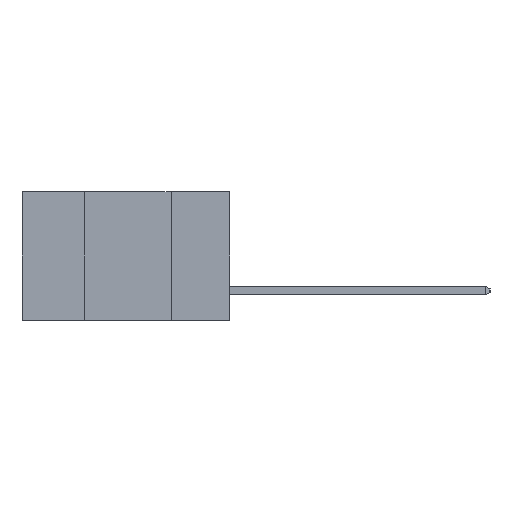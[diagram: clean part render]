
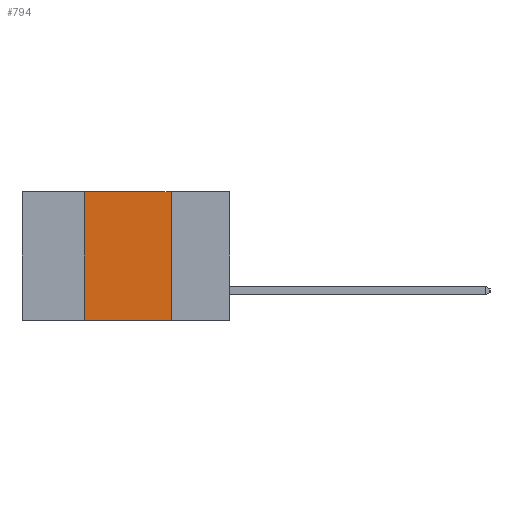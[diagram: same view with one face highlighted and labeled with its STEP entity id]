
A CAD part, left-side view. The second image highlights one B-rep face of the part: STEP entity #794.
In plain terms, the highlighted planar face has unit normal (-1, 0, 0).
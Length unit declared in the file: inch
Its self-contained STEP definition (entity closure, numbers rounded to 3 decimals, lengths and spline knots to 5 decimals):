
#26 = CARTESIAN_POINT ( 'NONE',  ( 0., 0.6, 0. ) ) ;
#627 = DIRECTION ( 'NONE',  ( 0., 0., -1. ) ) ;
#794 = ADVANCED_FACE ( 'NONE', ( #10889 ), #2431, .F. ) ;
#1288 = ORIENTED_EDGE ( 'NONE', *, *, #10157, .F. ) ;
#1415 = DIRECTION ( 'NONE',  ( 0., 0., 1. ) ) ;
#2431 = PLANE ( 'NONE',  #8279 ) ;
#2713 = LINE ( 'NONE', #5776, #10181 ) ;
#2920 = LINE ( 'NONE', #11767, #10082 ) ;
#3442 = VECTOR ( 'NONE', #8856, 39.37008 ) ;
#3503 = DIRECTION ( 'NONE',  ( 1., 0., 0. ) ) ;
#3769 = LINE ( 'NONE', #26, #3442 ) ;
#3923 = EDGE_LOOP ( 'NONE', ( #1288, #9534, #12179, #10366 ) ) ;
#3983 = VECTOR ( 'NONE', #1415, 39.37008 ) ;
#4303 = VERTEX_POINT ( 'NONE', #6328 ) ;
#4814 = CARTESIAN_POINT ( 'NONE',  ( 0., 0.6, 0. ) ) ;
#5368 = CARTESIAN_POINT ( 'NONE',  ( 0., 0.17, 0. ) ) ;
#5492 = VERTEX_POINT ( 'NONE', #7036 ) ;
#5776 = CARTESIAN_POINT ( 'NONE',  ( 0., 0.17, 0. ) ) ;
#6235 = LINE ( 'NONE', #7287, #3983 ) ;
#6251 = VERTEX_POINT ( 'NONE', #5368 ) ;
#6328 = CARTESIAN_POINT ( 'NONE',  ( 0., 0.42, -0.37 ) ) ;
#6390 = VERTEX_POINT ( 'NONE', #9241 ) ;
#6923 = EDGE_CURVE ( 'NONE', #4303, #5492, #6235, .T. ) ;
#7036 = CARTESIAN_POINT ( 'NONE',  ( 0., 0.42, 0. ) ) ;
#7234 = EDGE_CURVE ( 'NONE', #5492, #6251, #3769, .T. ) ;
#7287 = CARTESIAN_POINT ( 'NONE',  ( 0., 0.42, 0. ) ) ;
#8279 = AXIS2_PLACEMENT_3D ( 'NONE', #4814, #3503, #627 ) ;
#8749 = EDGE_CURVE ( 'NONE', #4303, #6390, #2920, .T. ) ;
#8856 = DIRECTION ( 'NONE',  ( 0., -1., 0. ) ) ;
#9137 = DIRECTION ( 'NONE',  ( 0., -1., 0. ) ) ;
#9241 = CARTESIAN_POINT ( 'NONE',  ( 0., 0.17, -0.37 ) ) ;
#9534 = ORIENTED_EDGE ( 'NONE', *, *, #7234, .F. ) ;
#10082 = VECTOR ( 'NONE', #9137, 39.37008 ) ;
#10157 = EDGE_CURVE ( 'NONE', #6251, #6390, #2713, .T. ) ;
#10181 = VECTOR ( 'NONE', #12072, 39.37008 ) ;
#10366 = ORIENTED_EDGE ( 'NONE', *, *, #8749, .T. ) ;
#10889 = FACE_OUTER_BOUND ( 'NONE', #3923, .T. ) ;
#11767 = CARTESIAN_POINT ( 'NONE',  ( 0., 0.6, -0.37 ) ) ;
#12072 = DIRECTION ( 'NONE',  ( 0., 0., -1. ) ) ;
#12179 = ORIENTED_EDGE ( 'NONE', *, *, #6923, .F. ) ;
